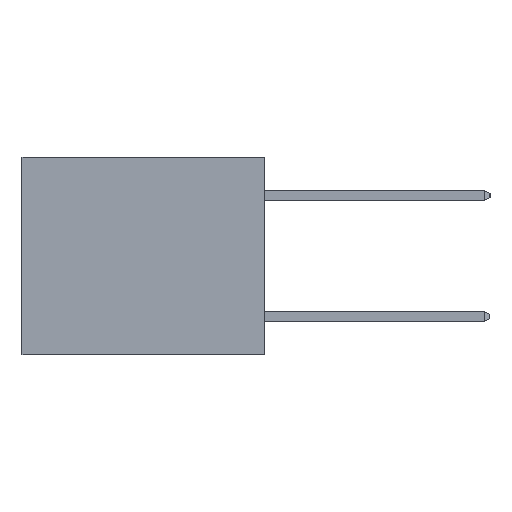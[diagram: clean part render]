
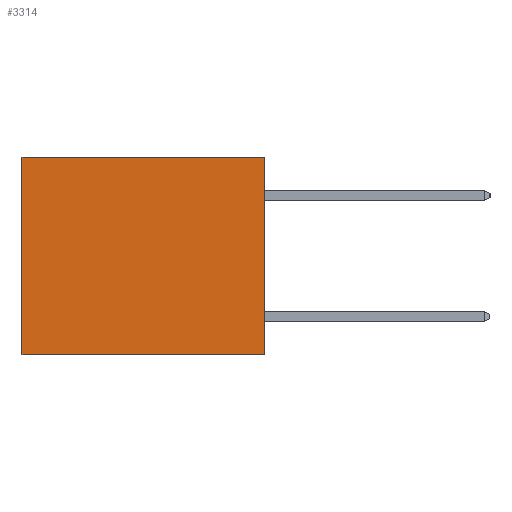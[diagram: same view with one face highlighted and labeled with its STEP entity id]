
A CAD part, left-side view. The second image highlights one B-rep face of the part: STEP entity #3314.
In plain terms, the highlighted planar face has unit normal (-1, 0, 0).
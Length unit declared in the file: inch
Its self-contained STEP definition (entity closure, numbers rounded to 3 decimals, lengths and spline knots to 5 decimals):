
#438 = VECTOR ( 'NONE', #4555, 39.37008 ) ;
#909 = LINE ( 'NONE', #7583, #438 ) ;
#1108 = LINE ( 'NONE', #9966, #17647 ) ;
#1325 = CARTESIAN_POINT ( 'NONE',  ( 0.3165, 0., -0.49 ) ) ;
#2353 = ORIENTED_EDGE ( 'NONE', *, *, #15770, .T. ) ;
#3016 = CARTESIAN_POINT ( 'NONE',  ( 0.3165, 0., -0.49 ) ) ;
#3078 = AXIS2_PLACEMENT_3D ( 'NONE', #1325, #13589, #16379 ) ;
#3314 = ADVANCED_FACE ( 'NONE', ( #4453 ), #18184, .F. ) ;
#4120 = CARTESIAN_POINT ( 'NONE',  ( 0.3165, 0.6, -0.49 ) ) ;
#4453 = FACE_OUTER_BOUND ( 'NONE', #9002, .T. ) ;
#4555 = DIRECTION ( 'NONE',  ( 0., 0., -1. ) ) ;
#4871 = CARTESIAN_POINT ( 'NONE',  ( 0.3165, 0., -0.49 ) ) ;
#5106 = LINE ( 'NONE', #5499, #6725 ) ;
#5160 = CARTESIAN_POINT ( 'NONE',  ( 0.3165, 0.6, 0. ) ) ;
#5204 = EDGE_CURVE ( 'NONE', #9737, #14440, #1108, .T. ) ;
#5316 = DIRECTION ( 'NONE',  ( 0., 1., 0. ) ) ;
#5499 = CARTESIAN_POINT ( 'NONE',  ( 0.3165, 0., 0. ) ) ;
#5679 = ORIENTED_EDGE ( 'NONE', *, *, #5204, .F. ) ;
#5829 = EDGE_CURVE ( 'NONE', #14408, #13169, #5106, .T. ) ;
#6059 = DIRECTION ( 'NONE',  ( 0., 0., -1. ) ) ;
#6725 = VECTOR ( 'NONE', #13676, 39.37008 ) ;
#7583 = CARTESIAN_POINT ( 'NONE',  ( 0.3165, 0.6, -0.49 ) ) ;
#8009 = ORIENTED_EDGE ( 'NONE', *, *, #5829, .T. ) ;
#9002 = EDGE_LOOP ( 'NONE', ( #2353, #5679, #13808, #8009 ) ) ;
#9737 = VERTEX_POINT ( 'NONE', #4871 ) ;
#9966 = CARTESIAN_POINT ( 'NONE',  ( 0.3165, 0., -0.49 ) ) ;
#11010 = LINE ( 'NONE', #3016, #14072 ) ;
#12168 = EDGE_CURVE ( 'NONE', #14408, #9737, #11010, .T. ) ;
#13169 = VERTEX_POINT ( 'NONE', #5160 ) ;
#13172 = CARTESIAN_POINT ( 'NONE',  ( 0.3165, 0., 0. ) ) ;
#13589 = DIRECTION ( 'NONE',  ( 1., 0., 0. ) ) ;
#13676 = DIRECTION ( 'NONE',  ( 0., 1., 0. ) ) ;
#13808 = ORIENTED_EDGE ( 'NONE', *, *, #12168, .F. ) ;
#14072 = VECTOR ( 'NONE', #6059, 39.37008 ) ;
#14408 = VERTEX_POINT ( 'NONE', #13172 ) ;
#14440 = VERTEX_POINT ( 'NONE', #4120 ) ;
#15770 = EDGE_CURVE ( 'NONE', #13169, #14440, #909, .T. ) ;
#16379 = DIRECTION ( 'NONE',  ( 0., 0., -1. ) ) ;
#17647 = VECTOR ( 'NONE', #5316, 39.37008 ) ;
#18184 = PLANE ( 'NONE',  #3078 ) ;
